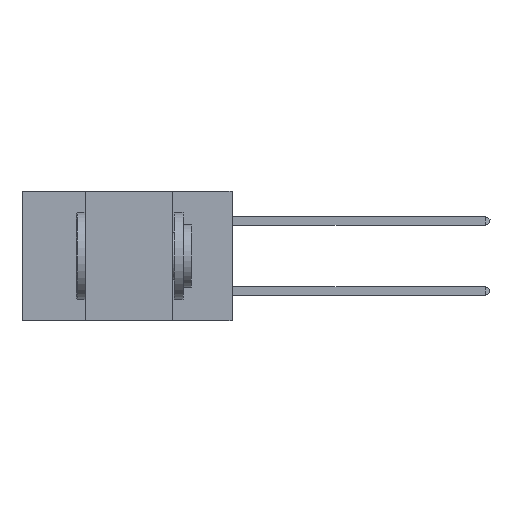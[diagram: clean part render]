
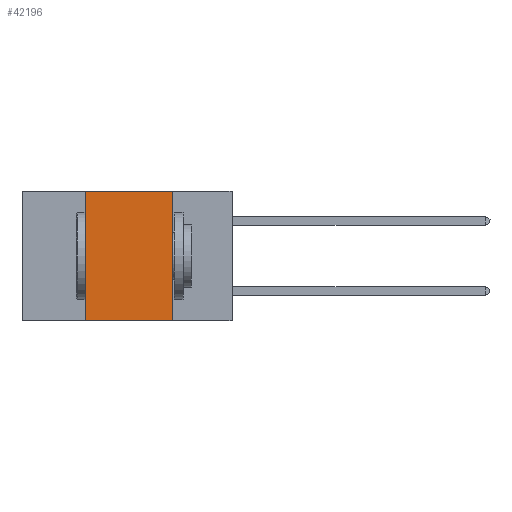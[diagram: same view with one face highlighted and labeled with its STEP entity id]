
A CAD part, left-side view. The second image highlights one B-rep face of the part: STEP entity #42196.
In plain terms, the highlighted planar face has unit normal (-1, 0, 0).
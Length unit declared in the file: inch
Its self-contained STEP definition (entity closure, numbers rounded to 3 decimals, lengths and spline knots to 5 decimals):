
#1205 = EDGE_CURVE ( 'NONE', #24620, #12737, #43177, .T. ) ;
#1372 = EDGE_CURVE ( 'NONE', #32357, #28162, #25072, .T. ) ;
#3501 = DIRECTION ( 'NONE',  ( 0., -1., 0. ) ) ;
#3856 = CARTESIAN_POINT ( 'NONE',  ( 0., 0.6, -0.37 ) ) ;
#5433 = FACE_OUTER_BOUND ( 'NONE', #12442, .T. ) ;
#6215 = ORIENTED_EDGE ( 'NONE', *, *, #1372, .F. ) ;
#8586 = CARTESIAN_POINT ( 'NONE',  ( 0., 0.6, 0. ) ) ;
#10831 = VECTOR ( 'NONE', #3501, 39.37008 ) ;
#11107 = VECTOR ( 'NONE', #41555, 39.37008 ) ;
#12442 = EDGE_LOOP ( 'NONE', ( #26206, #6215, #41662, #27706 ) ) ;
#12737 = VERTEX_POINT ( 'NONE', #44446 ) ;
#14928 = CARTESIAN_POINT ( 'NONE',  ( 0., 0.42, 0. ) ) ;
#15533 = LINE ( 'NONE', #41397, #11107 ) ;
#16014 = CARTESIAN_POINT ( 'NONE',  ( 0., 0.17, 0. ) ) ;
#17222 = DIRECTION ( 'NONE',  ( 0., -1., 0. ) ) ;
#18611 = VECTOR ( 'NONE', #17222, 39.37008 ) ;
#21229 = VECTOR ( 'NONE', #44694, 39.37008 ) ;
#23142 = DIRECTION ( 'NONE',  ( 0., 0., -1. ) ) ;
#23174 = EDGE_CURVE ( 'NONE', #28162, #12737, #15533, .T. ) ;
#23485 = LINE ( 'NONE', #41367, #21229 ) ;
#24620 = VERTEX_POINT ( 'NONE', #43567 ) ;
#25072 = LINE ( 'NONE', #8586, #10831 ) ;
#25974 = EDGE_CURVE ( 'NONE', #24620, #32357, #23485, .T. ) ;
#26206 = ORIENTED_EDGE ( 'NONE', *, *, #23174, .F. ) ;
#27706 = ORIENTED_EDGE ( 'NONE', *, *, #1205, .T. ) ;
#28162 = VERTEX_POINT ( 'NONE', #16014 ) ;
#32357 = VERTEX_POINT ( 'NONE', #14928 ) ;
#33400 = CARTESIAN_POINT ( 'NONE',  ( 0., 0.6, 0. ) ) ;
#33542 = PLANE ( 'NONE',  #38918 ) ;
#34298 = DIRECTION ( 'NONE',  ( 1., 0., 0. ) ) ;
#38918 = AXIS2_PLACEMENT_3D ( 'NONE', #33400, #34298, #23142 ) ;
#41367 = CARTESIAN_POINT ( 'NONE',  ( 0., 0.42, 0. ) ) ;
#41397 = CARTESIAN_POINT ( 'NONE',  ( 0., 0.17, 0. ) ) ;
#41555 = DIRECTION ( 'NONE',  ( 0., 0., -1. ) ) ;
#41662 = ORIENTED_EDGE ( 'NONE', *, *, #25974, .F. ) ;
#42196 = ADVANCED_FACE ( 'NONE', ( #5433 ), #33542, .F. ) ;
#43177 = LINE ( 'NONE', #3856, #18611 ) ;
#43567 = CARTESIAN_POINT ( 'NONE',  ( 0., 0.42, -0.37 ) ) ;
#44446 = CARTESIAN_POINT ( 'NONE',  ( 0., 0.17, -0.37 ) ) ;
#44694 = DIRECTION ( 'NONE',  ( 0., 0., 1. ) ) ;
